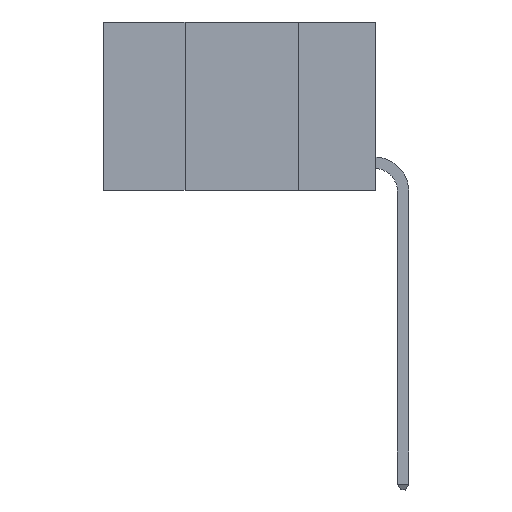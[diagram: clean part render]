
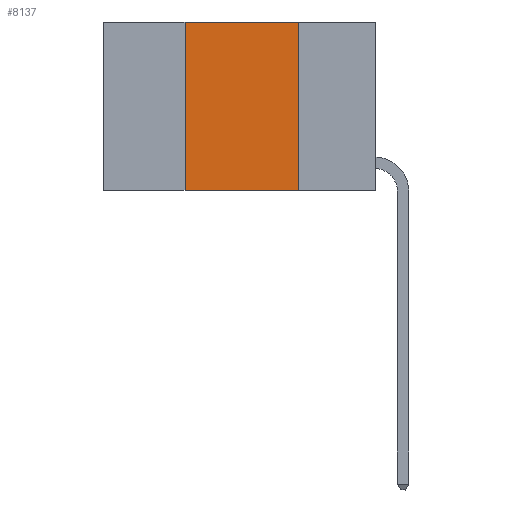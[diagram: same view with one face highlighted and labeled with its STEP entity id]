
A CAD part, left-side view. The second image highlights one B-rep face of the part: STEP entity #8137.
In plain terms, the highlighted planar face has unit normal (-1, 0, 0).
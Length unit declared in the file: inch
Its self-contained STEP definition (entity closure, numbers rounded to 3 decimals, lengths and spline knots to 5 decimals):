
#252 = DIRECTION ( 'NONE',  ( 0., 0., -1. ) ) ;
#768 = DIRECTION ( 'NONE',  ( 0., -1., 0. ) ) ;
#928 = VECTOR ( 'NONE', #27893, 39.37008 ) ;
#1538 = ORIENTED_EDGE ( 'NONE', *, *, #19640, .T. ) ;
#2382 = LINE ( 'NONE', #25705, #928 ) ;
#3148 = CARTESIAN_POINT ( 'NONE',  ( 0., 0.17, 0. ) ) ;
#4490 = EDGE_LOOP ( 'NONE', ( #28661, #11525, #18978, #1538 ) ) ;
#4574 = VECTOR ( 'NONE', #23545, 39.37008 ) ;
#4999 = CARTESIAN_POINT ( 'NONE',  ( 0., 0.17, -0.37 ) ) ;
#7749 = FACE_OUTER_BOUND ( 'NONE', #4490, .T. ) ;
#8137 = ADVANCED_FACE ( 'NONE', ( #7749 ), #25115, .F. ) ;
#9873 = VECTOR ( 'NONE', #768, 39.37008 ) ;
#10608 = LINE ( 'NONE', #12105, #28475 ) ;
#11525 = ORIENTED_EDGE ( 'NONE', *, *, #19649, .F. ) ;
#11632 = CARTESIAN_POINT ( 'NONE',  ( 0., 0.6, 0. ) ) ;
#12105 = CARTESIAN_POINT ( 'NONE',  ( 0., 0.6, -0.37 ) ) ;
#13876 = DIRECTION ( 'NONE',  ( 1., 0., 0. ) ) ;
#14062 = EDGE_CURVE ( 'NONE', #15331, #25916, #22635, .T. ) ;
#15331 = VERTEX_POINT ( 'NONE', #25311 ) ;
#16638 = LINE ( 'NONE', #16667, #9873 ) ;
#16667 = CARTESIAN_POINT ( 'NONE',  ( 0., 0.6, 0. ) ) ;
#18978 = ORIENTED_EDGE ( 'NONE', *, *, #22198, .F. ) ;
#19640 = EDGE_CURVE ( 'NONE', #23397, #25916, #10608, .T. ) ;
#19649 = EDGE_CURVE ( 'NONE', #20593, #15331, #16638, .T. ) ;
#20593 = VERTEX_POINT ( 'NONE', #27075 ) ;
#21370 = CARTESIAN_POINT ( 'NONE',  ( 0., 0.42, -0.37 ) ) ;
#22198 = EDGE_CURVE ( 'NONE', #23397, #20593, #2382, .T. ) ;
#22302 = AXIS2_PLACEMENT_3D ( 'NONE', #11632, #13876, #252 ) ;
#22635 = LINE ( 'NONE', #3148, #4574 ) ;
#23397 = VERTEX_POINT ( 'NONE', #21370 ) ;
#23545 = DIRECTION ( 'NONE',  ( 0., 0., -1. ) ) ;
#25115 = PLANE ( 'NONE',  #22302 ) ;
#25311 = CARTESIAN_POINT ( 'NONE',  ( 0., 0.17, 0. ) ) ;
#25600 = DIRECTION ( 'NONE',  ( 0., -1., 0. ) ) ;
#25705 = CARTESIAN_POINT ( 'NONE',  ( 0., 0.42, 0. ) ) ;
#25916 = VERTEX_POINT ( 'NONE', #4999 ) ;
#27075 = CARTESIAN_POINT ( 'NONE',  ( 0., 0.42, 0. ) ) ;
#27893 = DIRECTION ( 'NONE',  ( 0., 0., 1. ) ) ;
#28475 = VECTOR ( 'NONE', #25600, 39.37008 ) ;
#28661 = ORIENTED_EDGE ( 'NONE', *, *, #14062, .F. ) ;
